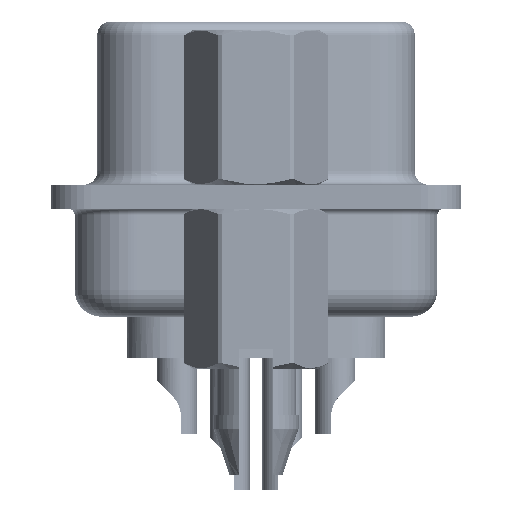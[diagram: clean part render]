
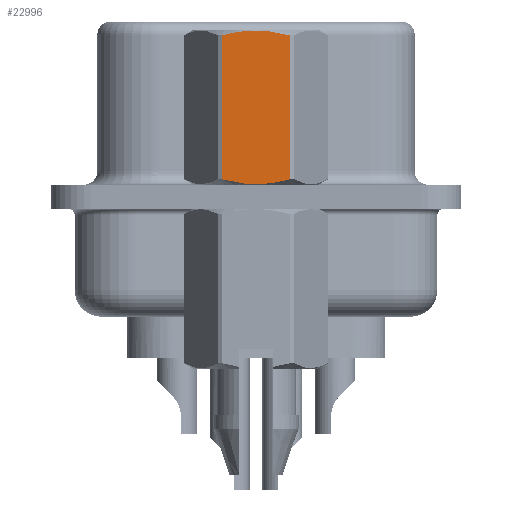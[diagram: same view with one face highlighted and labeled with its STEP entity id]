
A CAD part, left-side view. The second image highlights one B-rep face of the part: STEP entity #22996.
In plain terms, the highlighted planar face has unit normal (-1, 0, 0).
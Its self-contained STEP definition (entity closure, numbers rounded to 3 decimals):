
#244 = CARTESIAN_POINT ( 'NONE',  ( -2.381, -0.858, 6.15 ) ) ;
#1450 = ORIENTED_EDGE ( 'NONE', *, *, #39114, .T. ) ;
#2439 = DIRECTION ( 'NONE',  ( 0., 0., -1. ) ) ;
#2567 = CARTESIAN_POINT ( 'NONE',  ( -2.381, -0.215, 0.468 ) ) ;
#2891 = CARTESIAN_POINT ( 'NONE',  ( -2.381, 1.375, -3.75 ) ) ;
#4608 = CARTESIAN_POINT ( 'NONE',  ( -2.381, 1.273, 6.048 ) ) ;
#5151 = LINE ( 'NONE', #37428, #21465 ) ;
#5389 = CARTESIAN_POINT ( 'NONE',  ( -2.381, 0.215, 6.232 ) ) ;
#6170 = CARTESIAN_POINT ( 'NONE',  ( -2.381, 0.215, 0.468 ) ) ;
#7685 = CARTESIAN_POINT ( 'NONE',  ( -2.381, -0.215, 6.232 ) ) ;
#9793 = CARTESIAN_POINT ( 'NONE',  ( -2.381, 0.853, 0.549 ) ) ;
#9843 = CARTESIAN_POINT ( 'NONE',  ( -2.381, 1.273, 0.652 ) ) ;
#13981 = LINE ( 'NONE', #35638, #42942 ) ;
#14760 = B_SPLINE_CURVE_WITH_KNOTS ( 'NONE', 3,
 ( #18288, #21892, #244, #33673, #7685, #5389, #36349, #40413, #14897, #39934 ),
 .UNSPECIFIED., .F., .F.,
 ( 4, 2, 2, 2, 4 ),
 ( 0.001, 0.002, 0.002, 0.003, 0.004 ),
 .UNSPECIFIED. ) ;
#14795 = FACE_OUTER_BOUND ( 'NONE', #30131, .T. ) ;
#14897 = CARTESIAN_POINT ( 'NONE',  ( -2.381, 1.065, 6.104 ) ) ;
#18288 = CARTESIAN_POINT ( 'NONE',  ( -2.381, -1.273, 6.048 ) ) ;
#18553 = VERTEX_POINT ( 'NONE', #9843 ) ;
#20575 = ORIENTED_EDGE ( 'NONE', *, *, #32821, .T. ) ;
#21327 = CARTESIAN_POINT ( 'NONE',  ( -2.381, -0.432, 0.485 ) ) ;
#21465 = VECTOR ( 'NONE', #27306, 1000. ) ;
#21892 = CARTESIAN_POINT ( 'NONE',  ( -2.381, -1.066, 6.104 ) ) ;
#22996 = ADVANCED_FACE ( 'NONE', ( #14795 ), #30135, .T. ) ;
#24252 = CARTESIAN_POINT ( 'NONE',  ( -2.381, -0.858, 0.55 ) ) ;
#24488 = CARTESIAN_POINT ( 'NONE',  ( -2.381, 0.428, 0.485 ) ) ;
#25080 = VERTEX_POINT ( 'NONE', #33168 ) ;
#26005 = ORIENTED_EDGE ( 'NONE', *, *, #30591, .T. ) ;
#26397 = B_SPLINE_CURVE_WITH_KNOTS ( 'NONE', 3,
 ( #31462, #35068, #9793, #24488, #6170, #2567, #21327, #24252, #31930, #46610 ),
 .UNSPECIFIED., .F., .F.,
 ( 4, 2, 2, 2, 4 ),
 ( 0.003, 0.003, 0.004, 0.004, 0.005 ),
 .UNSPECIFIED. ) ;
#26601 = VERTEX_POINT ( 'NONE', #37380 ) ;
#27306 = DIRECTION ( 'NONE',  ( 0., 0., 1. ) ) ;
#27682 = AXIS2_PLACEMENT_3D ( 'NONE', #2891, #31794, #39483 ) ;
#30131 = EDGE_LOOP ( 'NONE', ( #41753, #20575, #26005, #1450 ) ) ;
#30135 = PLANE ( 'NONE',  #27682 ) ;
#30227 = VERTEX_POINT ( 'NONE', #4608 ) ;
#30591 = EDGE_CURVE ( 'NONE', #25080, #30227, #14760, .T. ) ;
#31462 = CARTESIAN_POINT ( 'NONE',  ( -2.381, 1.273, 0.652 ) ) ;
#31794 = DIRECTION ( 'NONE',  ( -1., 0., 0. ) ) ;
#31930 = CARTESIAN_POINT ( 'NONE',  ( -2.381, -1.066, 0.596 ) ) ;
#32821 = EDGE_CURVE ( 'NONE', #26601, #25080, #5151, .T. ) ;
#33168 = CARTESIAN_POINT ( 'NONE',  ( -2.381, -1.273, 6.048 ) ) ;
#33673 = CARTESIAN_POINT ( 'NONE',  ( -2.381, -0.432, 6.215 ) ) ;
#34996 = EDGE_CURVE ( 'NONE', #18553, #26601, #26397, .T. ) ;
#35068 = CARTESIAN_POINT ( 'NONE',  ( -2.381, 1.065, 0.596 ) ) ;
#35638 = CARTESIAN_POINT ( 'NONE',  ( -2.381, 1.273, 3.792 ) ) ;
#36349 = CARTESIAN_POINT ( 'NONE',  ( -2.381, 0.428, 6.215 ) ) ;
#37380 = CARTESIAN_POINT ( 'NONE',  ( -2.381, -1.273, 0.652 ) ) ;
#37428 = CARTESIAN_POINT ( 'NONE',  ( -2.381, -1.273, 3.792 ) ) ;
#39114 = EDGE_CURVE ( 'NONE', #30227, #18553, #13981, .T. ) ;
#39483 = DIRECTION ( 'NONE',  ( 0., -1., 0. ) ) ;
#39934 = CARTESIAN_POINT ( 'NONE',  ( -2.381, 1.273, 6.048 ) ) ;
#40413 = CARTESIAN_POINT ( 'NONE',  ( -2.381, 0.853, 6.151 ) ) ;
#41753 = ORIENTED_EDGE ( 'NONE', *, *, #34996, .T. ) ;
#42942 = VECTOR ( 'NONE', #2439, 1000. ) ;
#46610 = CARTESIAN_POINT ( 'NONE',  ( -2.381, -1.273, 0.652 ) ) ;
